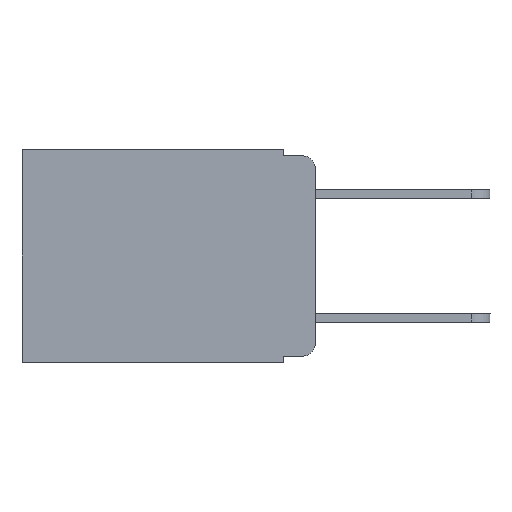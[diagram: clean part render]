
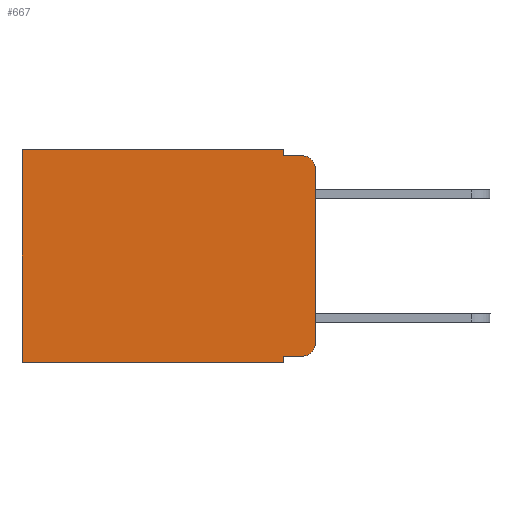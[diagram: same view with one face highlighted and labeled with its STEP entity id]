
A CAD part, left-side view. The second image highlights one B-rep face of the part: STEP entity #667.
In plain terms, the highlighted planar face has unit normal (-1, 0, 0).
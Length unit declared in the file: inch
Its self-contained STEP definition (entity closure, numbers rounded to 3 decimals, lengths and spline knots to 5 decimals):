
#73 = VERTEX_POINT ( 'NONE', #5983 ) ;
#279 = CARTESIAN_POINT ( 'NONE',  ( 0.298, 0.02, -0.333 ) ) ;
#282 = LINE ( 'NONE', #7591, #6601 ) ;
#366 = CARTESIAN_POINT ( 'NONE',  ( 0.298, 0.051, -0.333 ) ) ;
#606 = VERTEX_POINT ( 'NONE', #7483 ) ;
#667 = ADVANCED_FACE ( 'NONE', ( #2924 ), #10012, .F. ) ;
#706 = DIRECTION ( 'NONE',  ( 0., 0., -1. ) ) ;
#737 = CARTESIAN_POINT ( 'NONE',  ( 0.298, 0.051, 0. ) ) ;
#773 = DIRECTION ( 'NONE',  ( 0., 0., -1. ) ) ;
#1144 = AXIS2_PLACEMENT_3D ( 'NONE', #6067, #1467, #7793 ) ;
#1195 = VERTEX_POINT ( 'NONE', #8885 ) ;
#1215 = ORIENTED_EDGE ( 'NONE', *, *, #8724, .T. ) ;
#1221 = VECTOR ( 'NONE', #6460, 39.37008 ) ;
#1309 = AXIS2_PLACEMENT_3D ( 'NONE', #2091, #9137, #9924 ) ;
#1421 = VECTOR ( 'NONE', #773, 39.37008 ) ;
#1467 = DIRECTION ( 'NONE',  ( 1., 0., 0. ) ) ;
#1806 = CARTESIAN_POINT ( 'NONE',  ( 0.298, 0.051, 0. ) ) ;
#1848 = LINE ( 'NONE', #7209, #5920 ) ;
#1976 = LINE ( 'NONE', #7327, #10143 ) ;
#2070 = LINE ( 'NONE', #9754, #1221 ) ;
#2081 = DIRECTION ( 'NONE',  ( 0., 1., 0. ) ) ;
#2091 = CARTESIAN_POINT ( 'NONE',  ( 0.298, 0.02, -0.03 ) ) ;
#2282 = CARTESIAN_POINT ( 'NONE',  ( 0.298, 0.02, -0.313 ) ) ;
#2349 = EDGE_CURVE ( 'NONE', #3905, #73, #7848, .T. ) ;
#2538 = EDGE_LOOP ( 'NONE', ( #5005, #7267, #8168, #3067, #7388, #4843, #3324, #6021, #1215, #3612 ) ) ;
#2552 = CARTESIAN_POINT ( 'NONE',  ( 0.298, 0.473, 0. ) ) ;
#2582 = DIRECTION ( 'NONE',  ( 0., 0., -1. ) ) ;
#2924 = FACE_OUTER_BOUND ( 'NONE', #2538, .T. ) ;
#2955 = CIRCLE ( 'NONE', #1309, 0.02 ) ;
#3002 = DIRECTION ( 'NONE',  ( -1., 0., 0. ) ) ;
#3067 = ORIENTED_EDGE ( 'NONE', *, *, #2349, .F. ) ;
#3136 = LINE ( 'NONE', #7717, #7367 ) ;
#3179 = VERTEX_POINT ( 'NONE', #4134 ) ;
#3195 = VECTOR ( 'NONE', #3993, 39.37008 ) ;
#3295 = DIRECTION ( 'NONE',  ( 0., 0., -1. ) ) ;
#3317 = EDGE_CURVE ( 'NONE', #73, #1195, #282, .T. ) ;
#3324 = ORIENTED_EDGE ( 'NONE', *, *, #5856, .F. ) ;
#3342 = AXIS2_PLACEMENT_3D ( 'NONE', #2282, #3002, #706 ) ;
#3541 = EDGE_CURVE ( 'NONE', #8200, #4656, #4681, .T. ) ;
#3612 = ORIENTED_EDGE ( 'NONE', *, *, #4356, .T. ) ;
#3905 = VERTEX_POINT ( 'NONE', #1806 ) ;
#3993 = DIRECTION ( 'NONE',  ( 0., -1., 0. ) ) ;
#4134 = CARTESIAN_POINT ( 'NONE',  ( 0.298, 0., -0.03 ) ) ;
#4318 = EDGE_CURVE ( 'NONE', #6662, #606, #1976, .T. ) ;
#4356 = EDGE_CURVE ( 'NONE', #7984, #7132, #9546, .T. ) ;
#4460 = CARTESIAN_POINT ( 'NONE',  ( 0.298, 0., -0.313 ) ) ;
#4651 = CARTESIAN_POINT ( 'NONE',  ( 0.298, 0.473, -0.343 ) ) ;
#4656 = VERTEX_POINT ( 'NONE', #4651 ) ;
#4681 = LINE ( 'NONE', #2552, #5840 ) ;
#4843 = ORIENTED_EDGE ( 'NONE', *, *, #3541, .T. ) ;
#5005 = ORIENTED_EDGE ( 'NONE', *, *, #8904, .F. ) ;
#5037 = LINE ( 'NONE', #7110, #3195 ) ;
#5840 = VECTOR ( 'NONE', #3295, 39.37008 ) ;
#5856 = EDGE_CURVE ( 'NONE', #606, #4656, #1848, .T. ) ;
#5920 = VECTOR ( 'NONE', #8032, 39.37008 ) ;
#5983 = CARTESIAN_POINT ( 'NONE',  ( 0.298, 0.051, -0.01 ) ) ;
#6021 = ORIENTED_EDGE ( 'NONE', *, *, #4318, .F. ) ;
#6067 = CARTESIAN_POINT ( 'NONE',  ( 0.298, 0., 0. ) ) ;
#6460 = DIRECTION ( 'NONE',  ( 0., 0., -1. ) ) ;
#6601 = VECTOR ( 'NONE', #8983, 39.37008 ) ;
#6662 = VERTEX_POINT ( 'NONE', #366 ) ;
#7110 = CARTESIAN_POINT ( 'NONE',  ( 0.298, 0.051, -0.333 ) ) ;
#7132 = VERTEX_POINT ( 'NONE', #4460 ) ;
#7209 = CARTESIAN_POINT ( 'NONE',  ( 0.298, 0., -0.343 ) ) ;
#7266 = CARTESIAN_POINT ( 'NONE',  ( 0.298, 0.473, 0. ) ) ;
#7267 = ORIENTED_EDGE ( 'NONE', *, *, #8452, .T. ) ;
#7327 = CARTESIAN_POINT ( 'NONE',  ( 0.298, 0.051, 0. ) ) ;
#7367 = VECTOR ( 'NONE', #2081, 39.37008 ) ;
#7388 = ORIENTED_EDGE ( 'NONE', *, *, #10188, .T. ) ;
#7483 = CARTESIAN_POINT ( 'NONE',  ( 0.298, 0.051, -0.343 ) ) ;
#7591 = CARTESIAN_POINT ( 'NONE',  ( 0.298, 0.051, -0.01 ) ) ;
#7717 = CARTESIAN_POINT ( 'NONE',  ( 0.298, 0., 0. ) ) ;
#7793 = DIRECTION ( 'NONE',  ( 0., 0., -1. ) ) ;
#7848 = LINE ( 'NONE', #737, #1421 ) ;
#7984 = VERTEX_POINT ( 'NONE', #279 ) ;
#8032 = DIRECTION ( 'NONE',  ( 0., 1., 0. ) ) ;
#8168 = ORIENTED_EDGE ( 'NONE', *, *, #3317, .F. ) ;
#8200 = VERTEX_POINT ( 'NONE', #7266 ) ;
#8452 = EDGE_CURVE ( 'NONE', #3179, #1195, #2955, .T. ) ;
#8724 = EDGE_CURVE ( 'NONE', #6662, #7984, #5037, .T. ) ;
#8885 = CARTESIAN_POINT ( 'NONE',  ( 0.298, 0.02, -0.01 ) ) ;
#8904 = EDGE_CURVE ( 'NONE', #3179, #7132, #2070, .T. ) ;
#8983 = DIRECTION ( 'NONE',  ( 0., -1., 0. ) ) ;
#9137 = DIRECTION ( 'NONE',  ( -1., 0., 0. ) ) ;
#9546 = CIRCLE ( 'NONE', #3342, 0.02 ) ;
#9754 = CARTESIAN_POINT ( 'NONE',  ( 0.298, 0., 0. ) ) ;
#9924 = DIRECTION ( 'NONE',  ( 0., 0., -1. ) ) ;
#10012 = PLANE ( 'NONE',  #1144 ) ;
#10143 = VECTOR ( 'NONE', #2582, 39.37008 ) ;
#10188 = EDGE_CURVE ( 'NONE', #3905, #8200, #3136, .T. ) ;
